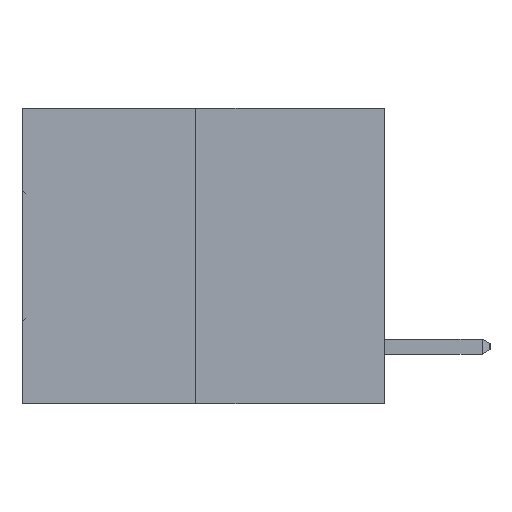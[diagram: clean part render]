
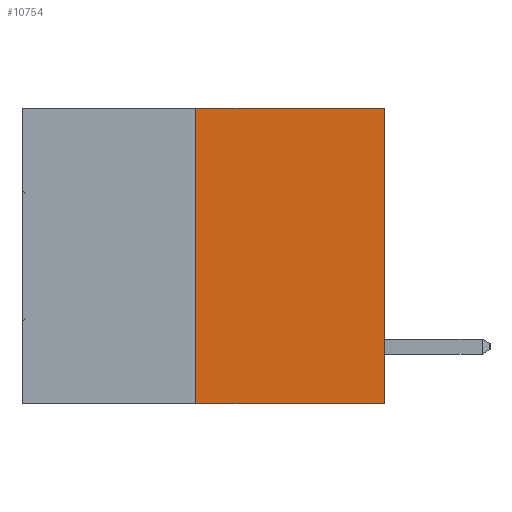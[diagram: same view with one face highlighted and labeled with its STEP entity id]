
A CAD part, left-side view. The second image highlights one B-rep face of the part: STEP entity #10754.
In plain terms, the highlighted planar face has unit normal (-1, 0, 0).
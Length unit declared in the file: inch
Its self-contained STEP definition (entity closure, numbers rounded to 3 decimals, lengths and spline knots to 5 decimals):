
#1701 = EDGE_CURVE ( 'NONE', #9698, #10145, #28791, .T. ) ;
#2424 = DIRECTION ( 'NONE',  ( 0., 0., -1. ) ) ;
#2452 = LINE ( 'NONE', #10617, #7830 ) ;
#2641 = CARTESIAN_POINT ( 'NONE',  ( 0., 0.6, 0. ) ) ;
#2760 = PLANE ( 'NONE',  #22710 ) ;
#3461 = EDGE_CURVE ( 'NONE', #24844, #9698, #26177, .T. ) ;
#5548 = ORIENTED_EDGE ( 'NONE', *, *, #3461, .T. ) ;
#6151 = VECTOR ( 'NONE', #8218, 39.37008 ) ;
#7815 = VECTOR ( 'NONE', #19196, 39.37008 ) ;
#7830 = VECTOR ( 'NONE', #31307, 39.37008 ) ;
#8218 = DIRECTION ( 'NONE',  ( 0., 0., 1. ) ) ;
#8447 = CARTESIAN_POINT ( 'NONE',  ( 0., 0.312, -0.49 ) ) ;
#8936 = CARTESIAN_POINT ( 'NONE',  ( 0., 0., -0.49 ) ) ;
#9698 = VERTEX_POINT ( 'NONE', #8936 ) ;
#9962 = ORIENTED_EDGE ( 'NONE', *, *, #14222, .F. ) ;
#10108 = FACE_OUTER_BOUND ( 'NONE', #11211, .T. ) ;
#10145 = VERTEX_POINT ( 'NONE', #10481 ) ;
#10481 = CARTESIAN_POINT ( 'NONE',  ( 0., 0., 0. ) ) ;
#10617 = CARTESIAN_POINT ( 'NONE',  ( 0., 0.6, 0. ) ) ;
#10741 = CARTESIAN_POINT ( 'NONE',  ( 0., 0.312, 0. ) ) ;
#10754 = ADVANCED_FACE ( 'NONE', ( #10108 ), #2760, .F. ) ;
#11211 = EDGE_LOOP ( 'NONE', ( #22396, #5548, #33241, #9962 ) ) ;
#12601 = VECTOR ( 'NONE', #24344, 39.37008 ) ;
#14222 = EDGE_CURVE ( 'NONE', #24706, #10145, #2452, .T. ) ;
#14257 = CARTESIAN_POINT ( 'NONE',  ( 0., 0.6, -0.49 ) ) ;
#15561 = DIRECTION ( 'NONE',  ( 1., 0., 0. ) ) ;
#19196 = DIRECTION ( 'NONE',  ( 0., 0., 1. ) ) ;
#21391 = LINE ( 'NONE', #8447, #6151 ) ;
#22396 = ORIENTED_EDGE ( 'NONE', *, *, #34085, .F. ) ;
#22710 = AXIS2_PLACEMENT_3D ( 'NONE', #2641, #15561, #2424 ) ;
#24344 = DIRECTION ( 'NONE',  ( 0., -1., 0. ) ) ;
#24706 = VERTEX_POINT ( 'NONE', #10741 ) ;
#24844 = VERTEX_POINT ( 'NONE', #30949 ) ;
#26177 = LINE ( 'NONE', #14257, #12601 ) ;
#28791 = LINE ( 'NONE', #29819, #7815 ) ;
#29819 = CARTESIAN_POINT ( 'NONE',  ( 0., 0., 0. ) ) ;
#30949 = CARTESIAN_POINT ( 'NONE',  ( 0., 0.312, -0.49 ) ) ;
#31307 = DIRECTION ( 'NONE',  ( 0., -1., 0. ) ) ;
#33241 = ORIENTED_EDGE ( 'NONE', *, *, #1701, .T. ) ;
#34085 = EDGE_CURVE ( 'NONE', #24844, #24706, #21391, .T. ) ;
